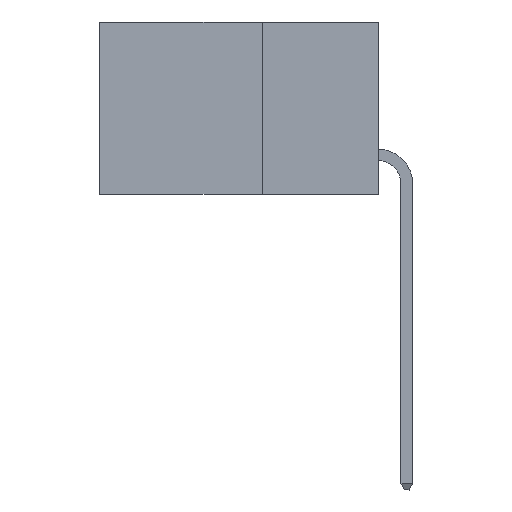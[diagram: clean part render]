
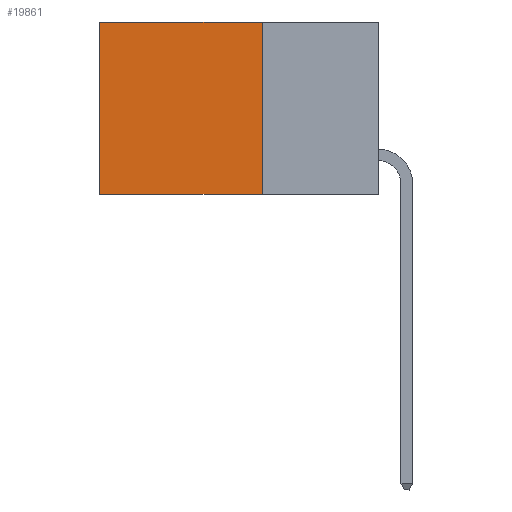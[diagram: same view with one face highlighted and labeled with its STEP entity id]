
A CAD part, left-side view. The second image highlights one B-rep face of the part: STEP entity #19861.
In plain terms, the highlighted planar face has unit normal (-1, 0, 0).
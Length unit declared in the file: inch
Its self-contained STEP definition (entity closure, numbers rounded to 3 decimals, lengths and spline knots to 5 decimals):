
#221 = LINE ( 'NONE', #19374, #8731 ) ;
#528 = FACE_OUTER_BOUND ( 'NONE', #4759, .T. ) ;
#707 = EDGE_CURVE ( 'NONE', #19189, #5006, #17827, .T. ) ;
#1408 = DIRECTION ( 'NONE',  ( 0., 0., -1. ) ) ;
#2203 = CARTESIAN_POINT ( 'NONE',  ( 0.298, 0.25, -0.37 ) ) ;
#2953 = DIRECTION ( 'NONE',  ( 0., 0., -1. ) ) ;
#4759 = EDGE_LOOP ( 'NONE', ( #10039, #5556, #19014, #20372 ) ) ;
#4918 = CARTESIAN_POINT ( 'NONE',  ( 0.298, 0.25, 0. ) ) ;
#5006 = VERTEX_POINT ( 'NONE', #13191 ) ;
#5556 = ORIENTED_EDGE ( 'NONE', *, *, #10269, .F. ) ;
#6472 = EDGE_CURVE ( 'NONE', #5006, #13925, #7682, .T. ) ;
#7119 = VECTOR ( 'NONE', #20151, 39.37008 ) ;
#7122 = CARTESIAN_POINT ( 'NONE',  ( 0.298, 0.25, -0.37 ) ) ;
#7682 = LINE ( 'NONE', #16854, #20180 ) ;
#8593 = VECTOR ( 'NONE', #9920, 39.37008 ) ;
#8731 = VECTOR ( 'NONE', #2953, 39.37008 ) ;
#9844 = PLANE ( 'NONE',  #10618 ) ;
#9920 = DIRECTION ( 'NONE',  ( 0., 1., 0. ) ) ;
#10039 = ORIENTED_EDGE ( 'NONE', *, *, #6472, .T. ) ;
#10269 = EDGE_CURVE ( 'NONE', #12010, #13925, #11455, .T. ) ;
#10484 = CARTESIAN_POINT ( 'NONE',  ( 0.298, 0.25, 0. ) ) ;
#10618 = AXIS2_PLACEMENT_3D ( 'NONE', #14770, #11517, #1408 ) ;
#11455 = LINE ( 'NONE', #7122, #7119 ) ;
#11517 = DIRECTION ( 'NONE',  ( 1., 0., 0. ) ) ;
#12010 = VERTEX_POINT ( 'NONE', #2203 ) ;
#13191 = CARTESIAN_POINT ( 'NONE',  ( 0.298, 0.6, 0. ) ) ;
#13925 = VERTEX_POINT ( 'NONE', #20358 ) ;
#14770 = CARTESIAN_POINT ( 'NONE',  ( 0.298, 0.25, 0. ) ) ;
#16854 = CARTESIAN_POINT ( 'NONE',  ( 0.298, 0.6, 0. ) ) ;
#16879 = DIRECTION ( 'NONE',  ( 0., 0., -1. ) ) ;
#17827 = LINE ( 'NONE', #10484, #8593 ) ;
#18425 = EDGE_CURVE ( 'NONE', #19189, #12010, #221, .T. ) ;
#19014 = ORIENTED_EDGE ( 'NONE', *, *, #18425, .F. ) ;
#19189 = VERTEX_POINT ( 'NONE', #4918 ) ;
#19374 = CARTESIAN_POINT ( 'NONE',  ( 0.298, 0.25, 0. ) ) ;
#19861 = ADVANCED_FACE ( 'NONE', ( #528 ), #9844, .F. ) ;
#20151 = DIRECTION ( 'NONE',  ( 0., 1., 0. ) ) ;
#20180 = VECTOR ( 'NONE', #16879, 39.37008 ) ;
#20358 = CARTESIAN_POINT ( 'NONE',  ( 0.298, 0.6, -0.37 ) ) ;
#20372 = ORIENTED_EDGE ( 'NONE', *, *, #707, .T. ) ;
